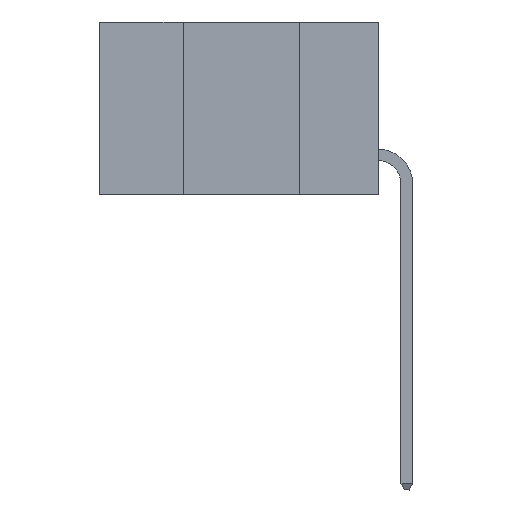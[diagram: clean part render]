
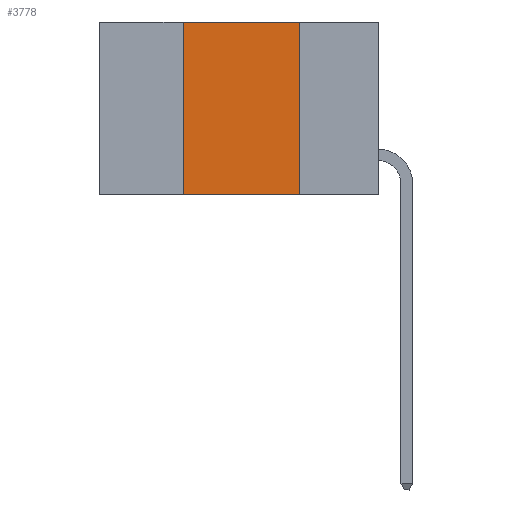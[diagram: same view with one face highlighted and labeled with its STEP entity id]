
A CAD part, left-side view. The second image highlights one B-rep face of the part: STEP entity #3778.
In plain terms, the highlighted planar face has unit normal (-1, 0, 0).
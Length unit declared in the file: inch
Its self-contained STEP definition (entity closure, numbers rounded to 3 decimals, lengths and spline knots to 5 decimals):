
#135 = CARTESIAN_POINT ( 'NONE',  ( 0., 0.42, 0. ) ) ;
#246 = CARTESIAN_POINT ( 'NONE',  ( 0., 0.6, 0. ) ) ;
#926 = DIRECTION ( 'NONE',  ( 0., 0., -1. ) ) ;
#1003 = ORIENTED_EDGE ( 'NONE', *, *, #9870, .F. ) ;
#1322 = DIRECTION ( 'NONE',  ( 0., 0., 1. ) ) ;
#2238 = CARTESIAN_POINT ( 'NONE',  ( 0., 0.6, 0. ) ) ;
#2412 = CARTESIAN_POINT ( 'NONE',  ( 0., 0.6, -0.37 ) ) ;
#2571 = LINE ( 'NONE', #2238, #8387 ) ;
#2717 = VERTEX_POINT ( 'NONE', #5102 ) ;
#3033 = DIRECTION ( 'NONE',  ( 1., 0., 0. ) ) ;
#3159 = VECTOR ( 'NONE', #1322, 39.37008 ) ;
#3442 = DIRECTION ( 'NONE',  ( 0., -1., 0. ) ) ;
#3778 = ADVANCED_FACE ( 'NONE', ( #5266 ), #7188, .F. ) ;
#3935 = LINE ( 'NONE', #2412, #9690 ) ;
#5024 = VERTEX_POINT ( 'NONE', #7077 ) ;
#5102 = CARTESIAN_POINT ( 'NONE',  ( 0., 0.42, -0.37 ) ) ;
#5266 = FACE_OUTER_BOUND ( 'NONE', #13479, .T. ) ;
#5570 = VECTOR ( 'NONE', #926, 39.37008 ) ;
#5970 = DIRECTION ( 'NONE',  ( 0., -1., 0. ) ) ;
#6038 = EDGE_CURVE ( 'NONE', #5024, #7990, #6272, .T. ) ;
#6272 = LINE ( 'NONE', #14633, #5570 ) ;
#6399 = VERTEX_POINT ( 'NONE', #8703 ) ;
#7077 = CARTESIAN_POINT ( 'NONE',  ( 0., 0.17, 0. ) ) ;
#7188 = PLANE ( 'NONE',  #11584 ) ;
#7990 = VERTEX_POINT ( 'NONE', #12875 ) ;
#8387 = VECTOR ( 'NONE', #3442, 39.37008 ) ;
#8703 = CARTESIAN_POINT ( 'NONE',  ( 0., 0.42, 0. ) ) ;
#9304 = LINE ( 'NONE', #135, #3159 ) ;
#9537 = ORIENTED_EDGE ( 'NONE', *, *, #6038, .F. ) ;
#9690 = VECTOR ( 'NONE', #5970, 39.37008 ) ;
#9870 = EDGE_CURVE ( 'NONE', #2717, #6399, #9304, .T. ) ;
#10528 = EDGE_CURVE ( 'NONE', #6399, #5024, #2571, .T. ) ;
#11584 = AXIS2_PLACEMENT_3D ( 'NONE', #246, #3033, #14873 ) ;
#12875 = CARTESIAN_POINT ( 'NONE',  ( 0., 0.17, -0.37 ) ) ;
#12895 = ORIENTED_EDGE ( 'NONE', *, *, #10528, .F. ) ;
#13234 = ORIENTED_EDGE ( 'NONE', *, *, #14356, .T. ) ;
#13479 = EDGE_LOOP ( 'NONE', ( #9537, #12895, #1003, #13234 ) ) ;
#14356 = EDGE_CURVE ( 'NONE', #2717, #7990, #3935, .T. ) ;
#14633 = CARTESIAN_POINT ( 'NONE',  ( 0., 0.17, 0. ) ) ;
#14873 = DIRECTION ( 'NONE',  ( 0., 0., -1. ) ) ;
